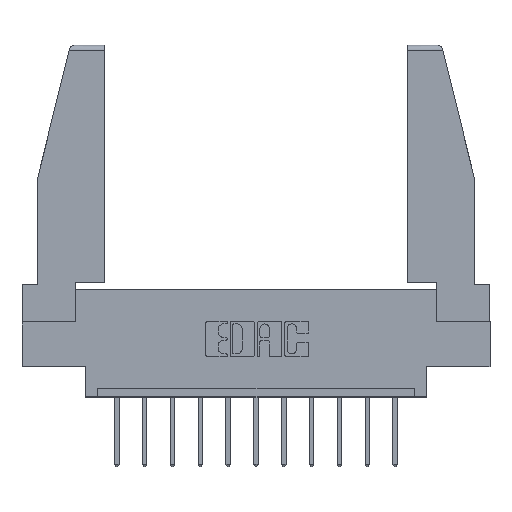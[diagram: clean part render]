
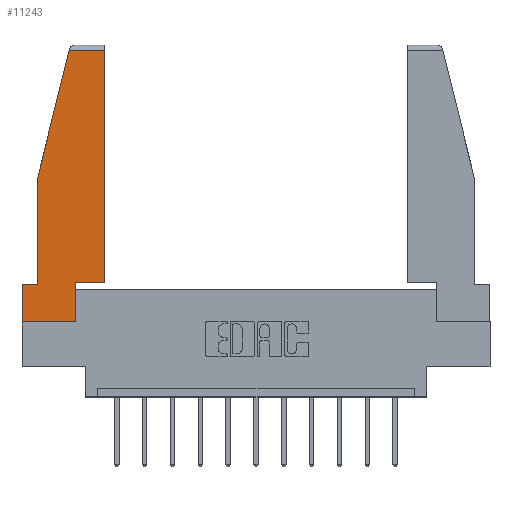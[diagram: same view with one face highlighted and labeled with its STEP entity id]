
A CAD part, top view. The second image highlights one B-rep face of the part: STEP entity #11243.
In plain terms, the highlighted planar face has unit normal (0, 0, 1).
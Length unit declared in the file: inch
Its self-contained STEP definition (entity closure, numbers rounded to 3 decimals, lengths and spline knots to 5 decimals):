
#20 = CARTESIAN_POINT ( 'NONE',  ( 0., 1.52, 0. ) ) ;
#53 = PLANE ( 'NONE',  #6156 ) ;
#217 = ORIENTED_EDGE ( 'NONE', *, *, #5587, .T. ) ;
#420 = LINE ( 'NONE', #4926, #9678 ) ;
#471 = CARTESIAN_POINT ( 'NONE',  ( 0.297, 0.223, 0. ) ) ;
#775 = VERTEX_POINT ( 'NONE', #1415 ) ;
#1155 = CARTESIAN_POINT ( 'NONE',  ( 0.297, 0., 0. ) ) ;
#1180 = CARTESIAN_POINT ( 'NONE',  ( 0., 0., 0. ) ) ;
#1399 = EDGE_CURVE ( 'NONE', #13309, #775, #4862, .T. ) ;
#1415 = CARTESIAN_POINT ( 'NONE',  ( 0., 0., 0. ) ) ;
#1446 = CARTESIAN_POINT ( 'NONE',  ( 0., 0.21, 0. ) ) ;
#1677 = VERTEX_POINT ( 'NONE', #14445 ) ;
#1720 = VERTEX_POINT ( 'NONE', #13130 ) ;
#1831 = VECTOR ( 'NONE', #8112, 39.37008 ) ;
#1837 = EDGE_CURVE ( 'NONE', #9508, #4302, #2168, .T. ) ;
#2043 = CARTESIAN_POINT ( 'NONE',  ( 0.297, 0.223, 0. ) ) ;
#2168 = LINE ( 'NONE', #2043, #12174 ) ;
#2456 = DIRECTION ( 'NONE',  ( 0., 0., 1. ) ) ;
#2471 = ORIENTED_EDGE ( 'NONE', *, *, #3389, .T. ) ;
#2516 = LINE ( 'NONE', #4079, #13773 ) ;
#2858 = ORIENTED_EDGE ( 'NONE', *, *, #7048, .T. ) ;
#2918 = VERTEX_POINT ( 'NONE', #8270 ) ;
#3265 = CARTESIAN_POINT ( 'NONE',  ( 0., 0.21, 0. ) ) ;
#3389 = EDGE_CURVE ( 'NONE', #775, #6511, #13749, .T. ) ;
#3502 = LINE ( 'NONE', #11596, #12610 ) ;
#3730 = DIRECTION ( 'NONE',  ( 0., 1., 0. ) ) ;
#3857 = LINE ( 'NONE', #7154, #5675 ) ;
#4010 = DIRECTION ( 'NONE',  ( 0., -1., 0. ) ) ;
#4079 = CARTESIAN_POINT ( 'NONE',  ( 0.271, 1.55, 0. ) ) ;
#4302 = VERTEX_POINT ( 'NONE', #4944 ) ;
#4354 = ORIENTED_EDGE ( 'NONE', *, *, #12380, .T. ) ;
#4749 = DIRECTION ( 'NONE',  ( 0., 1., 0. ) ) ;
#4862 = LINE ( 'NONE', #1446, #1831 ) ;
#4926 = CARTESIAN_POINT ( 'NONE',  ( 0.461, 0.223, 0. ) ) ;
#4944 = CARTESIAN_POINT ( 'NONE',  ( 0.461, 0.223, 0. ) ) ;
#5587 = EDGE_CURVE ( 'NONE', #2918, #11397, #7930, .T. ) ;
#5675 = VECTOR ( 'NONE', #11725, 39.37008 ) ;
#6156 = AXIS2_PLACEMENT_3D ( 'NONE', #1180, #2456, #12687 ) ;
#6335 = DIRECTION ( 'NONE',  ( -0.239, -0.971, 0. ) ) ;
#6511 = VERTEX_POINT ( 'NONE', #1155 ) ;
#7033 = VECTOR ( 'NONE', #4010, 39.37008 ) ;
#7048 = EDGE_CURVE ( 'NONE', #1677, #2918, #2516, .T. ) ;
#7154 = CARTESIAN_POINT ( 'NONE',  ( 0., 0.21, 0. ) ) ;
#7439 = ORIENTED_EDGE ( 'NONE', *, *, #1399, .T. ) ;
#7478 = CARTESIAN_POINT ( 'NONE',  ( 0.086, 0.8, 0. ) ) ;
#7930 = LINE ( 'NONE', #7478, #7033 ) ;
#8020 = DIRECTION ( 'NONE',  ( -1., 0., 0. ) ) ;
#8112 = DIRECTION ( 'NONE',  ( 0., -1., 0. ) ) ;
#8270 = CARTESIAN_POINT ( 'NONE',  ( 0.086, 0.8, 0. ) ) ;
#8276 = ORIENTED_EDGE ( 'NONE', *, *, #14030, .T. ) ;
#8349 = EDGE_LOOP ( 'NONE', ( #8592, #8276, #2858, #217, #10183, #7439, #2471, #4354, #13158 ) ) ;
#8485 = CARTESIAN_POINT ( 'NONE',  ( 0., 0., 0. ) ) ;
#8592 = ORIENTED_EDGE ( 'NONE', *, *, #10794, .T. ) ;
#9343 = EDGE_CURVE ( 'NONE', #11397, #13309, #3857, .T. ) ;
#9508 = VERTEX_POINT ( 'NONE', #471 ) ;
#9514 = DIRECTION ( 'NONE',  ( 1., 0., 0. ) ) ;
#9678 = VECTOR ( 'NONE', #3730, 39.37008 ) ;
#10183 = ORIENTED_EDGE ( 'NONE', *, *, #9343, .T. ) ;
#10634 = VECTOR ( 'NONE', #8020, 39.37008 ) ;
#10794 = EDGE_CURVE ( 'NONE', #4302, #1720, #420, .T. ) ;
#11074 = VECTOR ( 'NONE', #9514, 39.37008 ) ;
#11243 = ADVANCED_FACE ( 'NONE', ( #12284 ), #53, .T. ) ;
#11397 = VERTEX_POINT ( 'NONE', #14086 ) ;
#11596 = CARTESIAN_POINT ( 'NONE',  ( 0.297, 0., 0. ) ) ;
#11725 = DIRECTION ( 'NONE',  ( -1., 0., 0. ) ) ;
#12174 = VECTOR ( 'NONE', #13785, 39.37008 ) ;
#12284 = FACE_OUTER_BOUND ( 'NONE', #8349, .T. ) ;
#12380 = EDGE_CURVE ( 'NONE', #6511, #9508, #3502, .T. ) ;
#12610 = VECTOR ( 'NONE', #4749, 39.37008 ) ;
#12687 = DIRECTION ( 'NONE',  ( 1., 0., 0. ) ) ;
#13130 = CARTESIAN_POINT ( 'NONE',  ( 0.461, 1.52, 0. ) ) ;
#13158 = ORIENTED_EDGE ( 'NONE', *, *, #1837, .T. ) ;
#13309 = VERTEX_POINT ( 'NONE', #3265 ) ;
#13749 = LINE ( 'NONE', #8485, #11074 ) ;
#13773 = VECTOR ( 'NONE', #6335, 39.37008 ) ;
#13785 = DIRECTION ( 'NONE',  ( 1., 0., 0. ) ) ;
#14030 = EDGE_CURVE ( 'NONE', #1720, #1677, #14369, .T. ) ;
#14086 = CARTESIAN_POINT ( 'NONE',  ( 0.086, 0.21, 0. ) ) ;
#14369 = LINE ( 'NONE', #20, #10634 ) ;
#14445 = CARTESIAN_POINT ( 'NONE',  ( 0.2636, 1.52, 0. ) ) ;
